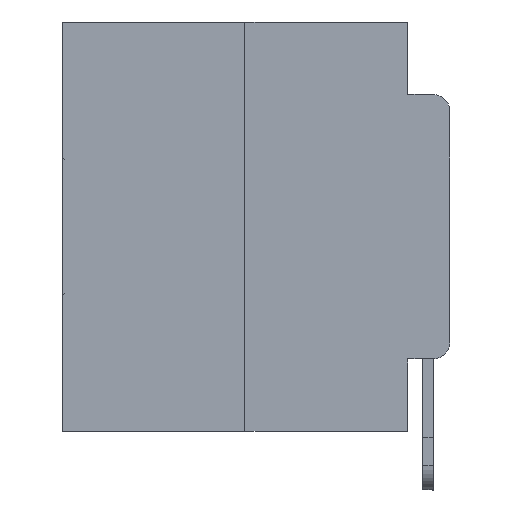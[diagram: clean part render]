
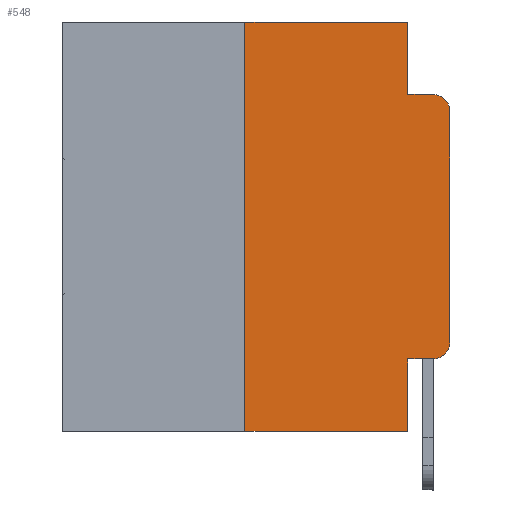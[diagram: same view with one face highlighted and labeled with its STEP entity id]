
A CAD part, left-side view. The second image highlights one B-rep face of the part: STEP entity #548.
In plain terms, the highlighted planar face has unit normal (-1, 0, 0).
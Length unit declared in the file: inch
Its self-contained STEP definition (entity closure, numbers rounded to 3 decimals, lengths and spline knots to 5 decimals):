
#180 = ORIENTED_EDGE ( 'NONE', *, *, #24556, .T. ) ;
#548 = ADVANCED_FACE ( 'NONE', ( #4959 ), #27876, .F. ) ;
#596 = CARTESIAN_POINT ( 'NONE',  ( 0., 0., -0.3915 ) ) ;
#1472 = AXIS2_PLACEMENT_3D ( 'NONE', #28460, #16912, #19450 ) ;
#2336 = CARTESIAN_POINT ( 'NONE',  ( 0., 0.25, 0. ) ) ;
#2545 = CARTESIAN_POINT ( 'NONE',  ( 0., 0., -0.1085 ) ) ;
#2660 = LINE ( 'NONE', #23012, #25011 ) ;
#2905 = EDGE_CURVE ( 'NONE', #11620, #18699, #21351, .T. ) ;
#3251 = CARTESIAN_POINT ( 'NONE',  ( 0., 0.473, -0.5 ) ) ;
#3394 = VERTEX_POINT ( 'NONE', #25823 ) ;
#3397 = DIRECTION ( 'NONE',  ( -1., 0., 0. ) ) ;
#3491 = DIRECTION ( 'NONE',  ( 0., 0., -1. ) ) ;
#3709 = DIRECTION ( 'NONE',  ( 0., 0., 1. ) ) ;
#4196 = VERTEX_POINT ( 'NONE', #5096 ) ;
#4440 = DIRECTION ( 'NONE',  ( 0., 0., 1. ) ) ;
#4959 = FACE_OUTER_BOUND ( 'NONE', #16225, .T. ) ;
#5096 = CARTESIAN_POINT ( 'NONE',  ( 0., 0.051, 0. ) ) ;
#5408 = ORIENTED_EDGE ( 'NONE', *, *, #8498, .F. ) ;
#6498 = EDGE_CURVE ( 'NONE', #15064, #4196, #27789, .T. ) ;
#7980 = CARTESIAN_POINT ( 'NONE',  ( 0., 0.051, -0.4115 ) ) ;
#8110 = AXIS2_PLACEMENT_3D ( 'NONE', #12802, #3397, #17313 ) ;
#8276 = CARTESIAN_POINT ( 'NONE',  ( 0., 0.051, 0. ) ) ;
#8498 = EDGE_CURVE ( 'NONE', #18869, #14749, #19442, .T. ) ;
#8871 = ORIENTED_EDGE ( 'NONE', *, *, #6498, .F. ) ;
#8994 = VECTOR ( 'NONE', #25674, 39.37008 ) ;
#9052 = LINE ( 'NONE', #2336, #28879 ) ;
#9248 = CARTESIAN_POINT ( 'NONE',  ( 0., 0.25, 0. ) ) ;
#9345 = CARTESIAN_POINT ( 'NONE',  ( 0., 0.473, 0. ) ) ;
#9351 = CARTESIAN_POINT ( 'NONE',  ( 0., 0.051, 0. ) ) ;
#10065 = VECTOR ( 'NONE', #21542, 39.37008 ) ;
#11620 = VERTEX_POINT ( 'NONE', #11795 ) ;
#11795 = CARTESIAN_POINT ( 'NONE',  ( 0., 0.25, -0.5 ) ) ;
#12566 = ORIENTED_EDGE ( 'NONE', *, *, #19494, .T. ) ;
#12768 = VERTEX_POINT ( 'NONE', #2545 ) ;
#12802 = CARTESIAN_POINT ( 'NONE',  ( 0., 0.02, -0.1085 ) ) ;
#12961 = VECTOR ( 'NONE', #3709, 39.37008 ) ;
#13348 = CIRCLE ( 'NONE', #8110, 0.02 ) ;
#14008 = DIRECTION ( 'NONE',  ( 0., -1., 0. ) ) ;
#14302 = DIRECTION ( 'NONE',  ( 0., -1., 0. ) ) ;
#14615 = VERTEX_POINT ( 'NONE', #596 ) ;
#14735 = ORIENTED_EDGE ( 'NONE', *, *, #17502, .F. ) ;
#14749 = VERTEX_POINT ( 'NONE', #28171 ) ;
#14904 = CARTESIAN_POINT ( 'NONE',  ( 0., 0., 0. ) ) ;
#15064 = VERTEX_POINT ( 'NONE', #9248 ) ;
#15141 = ORIENTED_EDGE ( 'NONE', *, *, #2905, .T. ) ;
#16225 = EDGE_LOOP ( 'NONE', ( #23134, #12566, #5408, #14735, #8871, #17574, #15141, #27061, #180, #29562 ) ) ;
#16907 = DIRECTION ( 'NONE',  ( 1., 0., 0. ) ) ;
#16912 = DIRECTION ( 'NONE',  ( -1., 0., 0. ) ) ;
#17313 = DIRECTION ( 'NONE',  ( 0., 0., -1. ) ) ;
#17502 = EDGE_CURVE ( 'NONE', #4196, #18869, #26848, .T. ) ;
#17574 = ORIENTED_EDGE ( 'NONE', *, *, #26185, .F. ) ;
#17682 = VECTOR ( 'NONE', #18780, 39.37008 ) ;
#18566 = EDGE_CURVE ( 'NONE', #21621, #18699, #23273, .T. ) ;
#18699 = VERTEX_POINT ( 'NONE', #19365 ) ;
#18780 = DIRECTION ( 'NONE',  ( 0., -1., 0. ) ) ;
#18869 = VERTEX_POINT ( 'NONE', #22945 ) ;
#19365 = CARTESIAN_POINT ( 'NONE',  ( 0., 0.051, -0.5 ) ) ;
#19442 = LINE ( 'NONE', #21396, #10065 ) ;
#19450 = DIRECTION ( 'NONE',  ( 0., 0., -1. ) ) ;
#19494 = EDGE_CURVE ( 'NONE', #12768, #14749, #13348, .T. ) ;
#20749 = VECTOR ( 'NONE', #14302, 39.37008 ) ;
#20841 = EDGE_CURVE ( 'NONE', #3394, #14615, #22506, .T. ) ;
#21105 = CARTESIAN_POINT ( 'NONE',  ( 0., 0.473, 0. ) ) ;
#21351 = LINE ( 'NONE', #3251, #20749 ) ;
#21381 = EDGE_CURVE ( 'NONE', #14615, #12768, #21657, .T. ) ;
#21396 = CARTESIAN_POINT ( 'NONE',  ( 0., 0.051, -0.0885 ) ) ;
#21542 = DIRECTION ( 'NONE',  ( 0., -1., 0. ) ) ;
#21621 = VERTEX_POINT ( 'NONE', #7980 ) ;
#21657 = LINE ( 'NONE', #14904, #12961 ) ;
#22506 = CIRCLE ( 'NONE', #1472, 0.02 ) ;
#22945 = CARTESIAN_POINT ( 'NONE',  ( 0., 0.051, -0.0885 ) ) ;
#23012 = CARTESIAN_POINT ( 'NONE',  ( 0., 0.051, -0.4115 ) ) ;
#23134 = ORIENTED_EDGE ( 'NONE', *, *, #21381, .T. ) ;
#23273 = LINE ( 'NONE', #9351, #8994 ) ;
#23797 = DIRECTION ( 'NONE',  ( 0., 0., -1. ) ) ;
#24556 = EDGE_CURVE ( 'NONE', #21621, #3394, #2660, .T. ) ;
#25011 = VECTOR ( 'NONE', #14008, 39.37008 ) ;
#25225 = VECTOR ( 'NONE', #3491, 39.37008 ) ;
#25478 = AXIS2_PLACEMENT_3D ( 'NONE', #21105, #16907, #23797 ) ;
#25674 = DIRECTION ( 'NONE',  ( 0., 0., -1. ) ) ;
#25823 = CARTESIAN_POINT ( 'NONE',  ( 0., 0.02, -0.4115 ) ) ;
#26185 = EDGE_CURVE ( 'NONE', #11620, #15064, #9052, .T. ) ;
#26848 = LINE ( 'NONE', #8276, #25225 ) ;
#27061 = ORIENTED_EDGE ( 'NONE', *, *, #18566, .F. ) ;
#27789 = LINE ( 'NONE', #9345, #17682 ) ;
#27876 = PLANE ( 'NONE',  #25478 ) ;
#28171 = CARTESIAN_POINT ( 'NONE',  ( 0., 0.02, -0.0885 ) ) ;
#28460 = CARTESIAN_POINT ( 'NONE',  ( 0., 0.02, -0.3915 ) ) ;
#28879 = VECTOR ( 'NONE', #4440, 39.37008 ) ;
#29562 = ORIENTED_EDGE ( 'NONE', *, *, #20841, .T. ) ;
